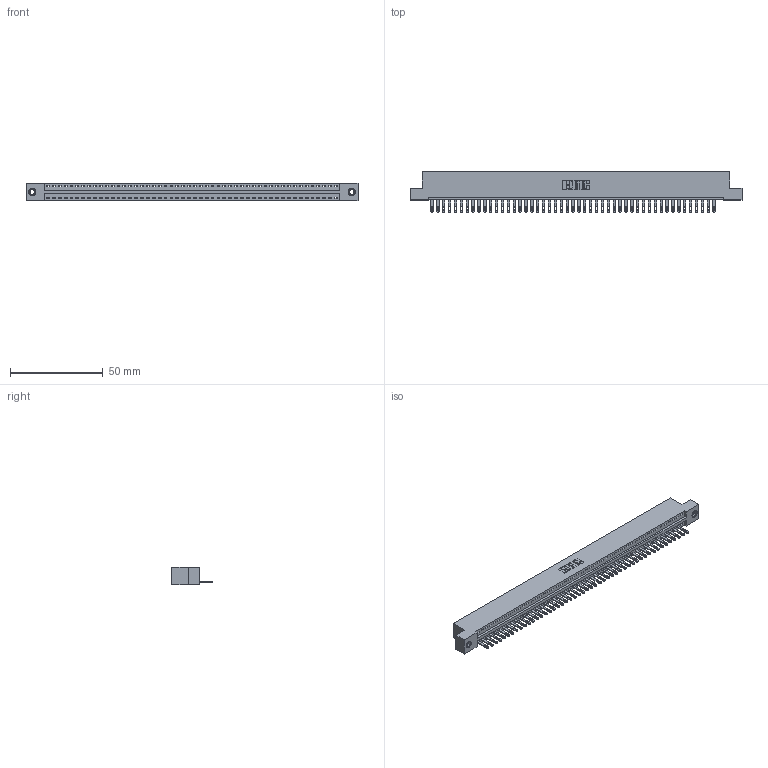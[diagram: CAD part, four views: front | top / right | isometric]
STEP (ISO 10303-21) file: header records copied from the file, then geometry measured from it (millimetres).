
FILE_DESCRIPTION (( 'STEP AP203' ), '1' );
FILE_NAME ('896-050-500-107.STEP', '2021-07-27T23:25:48', ( '' ), ( '' ), 'SwSTEP 2.0', 'SolidWorks 2020', '' );
FILE_SCHEMA (( 'CONFIG_CONTROL_DESIGN' ));
Length unit declared in the file: inch
Products named in the file (4): 896-050-500-107; 345-250-001_345-250-005-103; 846 Part_Flush Mounting Lugs - 0.156 Dia-TI; 345-292-001_345-293-100
Assembly tree (52 placements, depth 2):
  896-050-500-107
    846 Part_Flush Mounting Lugs - 0.156 Dia-TI
    345-292-001_345-293-100  x49
    345-250-001_345-250-005-103  x2
Bounding box: 179.32 x 21.84 x 9.4 mm (x, y, z)
Volume: 17225.8 mm3; surface area: 21703.6 mm2
Topology: 52 solids, 52 shells, 2840 faces, 8739 edges, 5818 vertices
Faces by surface type: plane 1784, cylinder 1040, cone 12, torus 4
Entity records: 31038 total; most frequent: CARTESIAN_POINT 5304, ORIENTED_EDGE 5282, DIRECTION 4697, EDGE_CURVE 2641, VECTOR 2285, LINE 2285, VERTEX_POINT 1756, AXIS2_PLACEMENT_3D 1206
